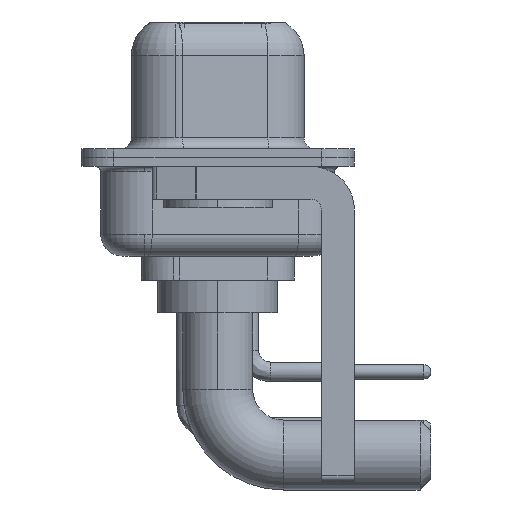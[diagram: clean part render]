
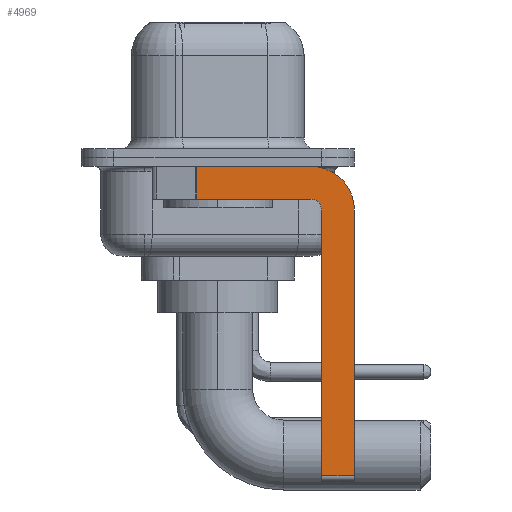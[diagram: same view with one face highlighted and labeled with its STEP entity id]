
A CAD part, left-side view. The second image highlights one B-rep face of the part: STEP entity #4969.
In plain terms, the highlighted planar face has unit normal (-1, 0, 0).
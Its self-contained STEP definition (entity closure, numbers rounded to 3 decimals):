
#265 = LINE ( 'NONE', #23256, #10550 ) ;
#372 = CARTESIAN_POINT ( 'NONE',  ( -2.9, -4.25, -1.9 ) ) ;
#389 = ORIENTED_EDGE ( 'NONE', *, *, #3927, .T. ) ;
#494 = CARTESIAN_POINT ( 'NONE',  ( -2.9, -4.75, -2.4 ) ) ;
#635 = LINE ( 'NONE', #12073, #11751 ) ;
#898 = EDGE_CURVE ( 'NONE', #17015, #23814, #635, .T. ) ;
#933 = EDGE_CURVE ( 'NONE', #17311, #17416, #265, .T. ) ;
#1202 = EDGE_CURVE ( 'NONE', #19927, #4610, #8566, .T. ) ;
#1343 = DIRECTION ( 'NONE',  ( 1., 0., 0. ) ) ;
#2138 = CARTESIAN_POINT ( 'NONE',  ( -2.9, -4.25, -0.4 ) ) ;
#2903 = CARTESIAN_POINT ( 'NONE',  ( -2.9, -6.25, -2.4 ) ) ;
#3927 = EDGE_CURVE ( 'NONE', #19927, #17416, #23658, .T. ) ;
#3982 = DIRECTION ( 'NONE',  ( 0., 0., -1. ) ) ;
#4610 = VERTEX_POINT ( 'NONE', #494 ) ;
#4723 = CIRCLE ( 'NONE', #20227, 0.5 ) ;
#4969 = ADVANCED_FACE ( 'NONE', ( #12545 ), #5314, .F. ) ;
#5314 = PLANE ( 'NONE',  #22364 ) ;
#5413 = CARTESIAN_POINT ( 'NONE',  ( -2.9, 0.978, -0.4 ) ) ;
#5480 = EDGE_LOOP ( 'NONE', ( #13532, #11271, #24078, #19384, #8095, #389, #20555, #8458 ) ) ;
#5902 = VERTEX_POINT ( 'NONE', #372 ) ;
#6604 = CARTESIAN_POINT ( 'NONE',  ( -2.9, -4.25, -14.55 ) ) ;
#7439 = CARTESIAN_POINT ( 'NONE',  ( -2.9, -4.75, -14.55 ) ) ;
#7994 = CARTESIAN_POINT ( 'NONE',  ( -2.9, 3., -0.4 ) ) ;
#8095 = ORIENTED_EDGE ( 'NONE', *, *, #1202, .F. ) ;
#8458 = ORIENTED_EDGE ( 'NONE', *, *, #9885, .F. ) ;
#8566 = LINE ( 'NONE', #16164, #10375 ) ;
#8908 = DIRECTION ( 'NONE',  ( 0., 0., -1. ) ) ;
#9133 = DIRECTION ( 'NONE',  ( 0., 1., 0. ) ) ;
#9885 = EDGE_CURVE ( 'NONE', #23553, #17311, #10978, .T. ) ;
#9938 = DIRECTION ( 'NONE',  ( -1., 0., 0. ) ) ;
#10375 = VECTOR ( 'NONE', #22741, 1000. ) ;
#10550 = VECTOR ( 'NONE', #23145, 1000. ) ;
#10674 = DIRECTION ( 'NONE',  ( 1., 0., 0. ) ) ;
#10978 = CIRCLE ( 'NONE', #15741, 2. ) ;
#11271 = ORIENTED_EDGE ( 'NONE', *, *, #898, .T. ) ;
#11691 = CARTESIAN_POINT ( 'NONE',  ( -2.9, -4.25, -2.4 ) ) ;
#11751 = VECTOR ( 'NONE', #3982, 1000. ) ;
#12073 = CARTESIAN_POINT ( 'NONE',  ( -2.9, 0.978, -1.9 ) ) ;
#12545 = FACE_OUTER_BOUND ( 'NONE', #5480, .T. ) ;
#12709 = CARTESIAN_POINT ( 'NONE',  ( -2.9, 0.978, -1.9 ) ) ;
#13532 = ORIENTED_EDGE ( 'NONE', *, *, #14657, .F. ) ;
#13730 = DIRECTION ( 'NONE',  ( 0., -1., 0. ) ) ;
#14657 = EDGE_CURVE ( 'NONE', #17015, #23553, #17458, .T. ) ;
#14845 = VECTOR ( 'NONE', #9133, 1000. ) ;
#15741 = AXIS2_PLACEMENT_3D ( 'NONE', #21850, #1343, #8908 ) ;
#16164 = CARTESIAN_POINT ( 'NONE',  ( -2.9, -4.75, -14.8 ) ) ;
#16203 = VECTOR ( 'NONE', #13730, 1000. ) ;
#16400 = DIRECTION ( 'NONE',  ( 0., 0., -1. ) ) ;
#16612 = LINE ( 'NONE', #20463, #14845 ) ;
#16894 = EDGE_CURVE ( 'NONE', #4610, #5902, #4723, .T. ) ;
#17015 = VERTEX_POINT ( 'NONE', #5413 ) ;
#17311 = VERTEX_POINT ( 'NONE', #2903 ) ;
#17416 = VERTEX_POINT ( 'NONE', #21574 ) ;
#17458 = LINE ( 'NONE', #7994, #16203 ) ;
#17531 = DIRECTION ( 'NONE',  ( 0., 0., 1. ) ) ;
#17933 = VECTOR ( 'NONE', #21923, 1000. ) ;
#19384 = ORIENTED_EDGE ( 'NONE', *, *, #16894, .F. ) ;
#19927 = VERTEX_POINT ( 'NONE', #7439 ) ;
#20227 = AXIS2_PLACEMENT_3D ( 'NONE', #11691, #9938, #17531 ) ;
#20463 = CARTESIAN_POINT ( 'NONE',  ( -2.9, -4.25, -1.9 ) ) ;
#20555 = ORIENTED_EDGE ( 'NONE', *, *, #933, .F. ) ;
#21574 = CARTESIAN_POINT ( 'NONE',  ( -2.9, -6.25, -14.55 ) ) ;
#21850 = CARTESIAN_POINT ( 'NONE',  ( -2.9, -4.25, -2.4 ) ) ;
#21923 = DIRECTION ( 'NONE',  ( 0., -1., 0. ) ) ;
#22291 = EDGE_CURVE ( 'NONE', #5902, #23814, #16612, .T. ) ;
#22364 = AXIS2_PLACEMENT_3D ( 'NONE', #24217, #10674, #16400 ) ;
#22741 = DIRECTION ( 'NONE',  ( 0., 0., 1. ) ) ;
#23145 = DIRECTION ( 'NONE',  ( 0., 0., -1. ) ) ;
#23256 = CARTESIAN_POINT ( 'NONE',  ( -2.9, -6.25, -2.4 ) ) ;
#23553 = VERTEX_POINT ( 'NONE', #2138 ) ;
#23658 = LINE ( 'NONE', #6604, #17933 ) ;
#23814 = VERTEX_POINT ( 'NONE', #12709 ) ;
#24078 = ORIENTED_EDGE ( 'NONE', *, *, #22291, .F. ) ;
#24217 = CARTESIAN_POINT ( 'NONE',  ( -2.9, -4.25, -2.4 ) ) ;
